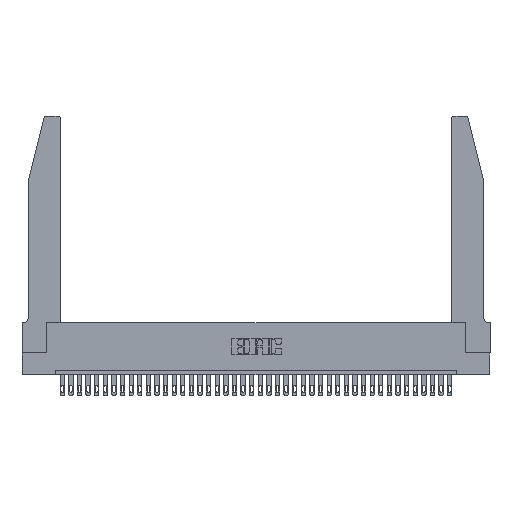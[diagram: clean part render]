
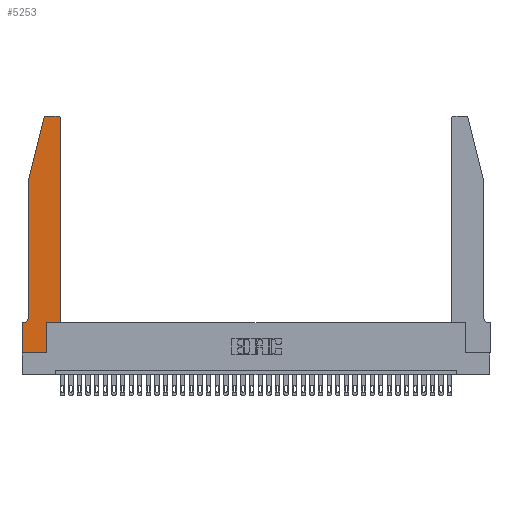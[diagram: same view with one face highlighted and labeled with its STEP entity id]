
A CAD part, top view. The second image highlights one B-rep face of the part: STEP entity #5253.
In plain terms, the highlighted planar face has unit normal (0, 0, 1).
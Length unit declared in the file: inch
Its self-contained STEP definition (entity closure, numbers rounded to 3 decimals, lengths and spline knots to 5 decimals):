
#120 = CARTESIAN_POINT ( 'NONE',  ( 0.2865, 0., 0.37 ) ) ;
#395 = CARTESIAN_POINT ( 'NONE',  ( 0.284, 2.75, 0.37 ) ) ;
#1014 = EDGE_CURVE ( 'NONE', #33882, #28112, #30752, .T. ) ;
#1118 = VERTEX_POINT ( 'NONE', #13074 ) ;
#1124 = LINE ( 'NONE', #24255, #33448 ) ;
#1738 = EDGE_CURVE ( 'NONE', #1118, #33882, #7715, .T. ) ;
#1933 = CARTESIAN_POINT ( 'NONE',  ( 0.2865, 0.35, 0.37 ) ) ;
#1951 = EDGE_LOOP ( 'NONE', ( #24118, #35103, #32265, #30136, #18198, #36965, #20821, #18857, #14239, #2538, #18210, #14275 ) ) ;
#2360 = DIRECTION ( 'NONE',  ( 0., 0., 1. ) ) ;
#2471 = DIRECTION ( 'NONE',  ( 0., -1., 0. ) ) ;
#2538 = ORIENTED_EDGE ( 'NONE', *, *, #29575, .T. ) ;
#2590 = LINE ( 'NONE', #33166, #35360 ) ;
#2778 = VERTEX_POINT ( 'NONE', #35461 ) ;
#3053 = VERTEX_POINT ( 'NONE', #3162 ) ;
#3073 = VECTOR ( 'NONE', #36618, 39.37008 ) ;
#3162 = CARTESIAN_POINT ( 'NONE',  ( 0.0055, 0.35, 0.37 ) ) ;
#3468 = EDGE_CURVE ( 'NONE', #3053, #14425, #10390, .T. ) ;
#3644 = DIRECTION ( 'NONE',  ( -1., 0., 0. ) ) ;
#4509 = CARTESIAN_POINT ( 'NONE',  ( 0.4205, 2.72, 0.37 ) ) ;
#4704 = DIRECTION ( 'NONE',  ( 1., 0., 0. ) ) ;
#5253 = ADVANCED_FACE ( 'NONE', ( #21943 ), #31846, .T. ) ;
#5536 = CARTESIAN_POINT ( 'NONE',  ( 0.2605, 2.75, 0.37 ) ) ;
#5701 = CARTESIAN_POINT ( 'NONE',  ( 0.4505, 0.35, 0.37 ) ) ;
#6025 = LINE ( 'NONE', #5701, #22372 ) ;
#7283 = AXIS2_PLACEMENT_3D ( 'NONE', #8476, #2360, #8876 ) ;
#7715 = LINE ( 'NONE', #5536, #3073 ) ;
#8432 = EDGE_CURVE ( 'NONE', #14425, #2778, #1124, .T. ) ;
#8476 = CARTESIAN_POINT ( 'NONE',  ( 0., 0.35, 0.37 ) ) ;
#8605 = VERTEX_POINT ( 'NONE', #27648 ) ;
#8876 = DIRECTION ( 'NONE',  ( 1., 0., 0. ) ) ;
#9354 = CARTESIAN_POINT ( 'NONE',  ( 0.4505, 2.72, 0.37 ) ) ;
#9806 = EDGE_CURVE ( 'NONE', #36554, #10278, #14082, .T. ) ;
#9826 = VERTEX_POINT ( 'NONE', #35048 ) ;
#10278 = VERTEX_POINT ( 'NONE', #28850 ) ;
#10390 = LINE ( 'NONE', #20717, #37070 ) ;
#10486 = DIRECTION ( 'NONE',  ( 0., 1., 0. ) ) ;
#11458 = DIRECTION ( 'NONE',  ( -1., 0., 0. ) ) ;
#11618 = VERTEX_POINT ( 'NONE', #19619 ) ;
#13074 = CARTESIAN_POINT ( 'NONE',  ( 0.4205, 2.75, 0.37 ) ) ;
#13326 = VECTOR ( 'NONE', #10486, 39.37008 ) ;
#13719 = DIRECTION ( 'NONE',  ( 0., 0., 1. ) ) ;
#14082 = LINE ( 'NONE', #1933, #17372 ) ;
#14101 = EDGE_CURVE ( 'NONE', #9826, #8605, #27517, .T. ) ;
#14239 = ORIENTED_EDGE ( 'NONE', *, *, #9806, .T. ) ;
#14275 = ORIENTED_EDGE ( 'NONE', *, *, #19880, .T. ) ;
#14425 = VERTEX_POINT ( 'NONE', #31439 ) ;
#15294 = EDGE_CURVE ( 'NONE', #2778, #36554, #2590, .T. ) ;
#16641 = LINE ( 'NONE', #32832, #21338 ) ;
#16779 = DIRECTION ( 'NONE',  ( 0., 0., 1. ) ) ;
#17372 = VECTOR ( 'NONE', #37898, 39.37008 ) ;
#18158 = CARTESIAN_POINT ( 'NONE',  ( 0.0055, 0.42, 0.37 ) ) ;
#18198 = ORIENTED_EDGE ( 'NONE', *, *, #27219, .T. ) ;
#18210 = ORIENTED_EDGE ( 'NONE', *, *, #33066, .T. ) ;
#18857 = ORIENTED_EDGE ( 'NONE', *, *, #15294, .T. ) ;
#19619 = CARTESIAN_POINT ( 'NONE',  ( 0.4505, 0.35, 0.37 ) ) ;
#19880 = EDGE_CURVE ( 'NONE', #29419, #1118, #32751, .T. ) ;
#20717 = CARTESIAN_POINT ( 'NONE',  ( 0.0755, 0.35, 0.37 ) ) ;
#20821 = ORIENTED_EDGE ( 'NONE', *, *, #8432, .T. ) ;
#21156 = EDGE_CURVE ( 'NONE', #28112, #9826, #16641, .T. ) ;
#21338 = VECTOR ( 'NONE', #30619, 39.37008 ) ;
#21943 = FACE_OUTER_BOUND ( 'NONE', #1951, .T. ) ;
#21995 = CARTESIAN_POINT ( 'NONE',  ( 0.284, 2.72, 0.37 ) ) ;
#22372 = VECTOR ( 'NONE', #29413, 39.37008 ) ;
#22540 = AXIS2_PLACEMENT_3D ( 'NONE', #18158, #27367, #3644 ) ;
#24118 = ORIENTED_EDGE ( 'NONE', *, *, #1738, .T. ) ;
#24255 = CARTESIAN_POINT ( 'NONE',  ( 0., 0., 0.37 ) ) ;
#25555 = DIRECTION ( 'NONE',  ( 1., 0., 0. ) ) ;
#25920 = CARTESIAN_POINT ( 'NONE',  ( 0.0755, 2., 0.37 ) ) ;
#26190 = DIRECTION ( 'NONE',  ( 0., -1., 0. ) ) ;
#27054 = VECTOR ( 'NONE', #26190, 39.37008 ) ;
#27219 = EDGE_CURVE ( 'NONE', #8605, #3053, #35181, .T. ) ;
#27367 = DIRECTION ( 'NONE',  ( 0., 0., -1. ) ) ;
#27517 = LINE ( 'NONE', #25920, #27054 ) ;
#27648 = CARTESIAN_POINT ( 'NONE',  ( 0.0755, 0.42, 0.37 ) ) ;
#28112 = VERTEX_POINT ( 'NONE', #38316 ) ;
#28827 = CARTESIAN_POINT ( 'NONE',  ( 0.4505, 0.35, 0.37 ) ) ;
#28850 = CARTESIAN_POINT ( 'NONE',  ( 0.2865, 0.35, 0.37 ) ) ;
#29358 = LINE ( 'NONE', #28827, #13326 ) ;
#29413 = DIRECTION ( 'NONE',  ( 1., 0., 0. ) ) ;
#29419 = VERTEX_POINT ( 'NONE', #9354 ) ;
#29575 = EDGE_CURVE ( 'NONE', #10278, #11618, #6025, .T. ) ;
#30136 = ORIENTED_EDGE ( 'NONE', *, *, #14101, .T. ) ;
#30452 = AXIS2_PLACEMENT_3D ( 'NONE', #4509, #16779, #31786 ) ;
#30619 = DIRECTION ( 'NONE',  ( -0.239, -0.971, 0. ) ) ;
#30752 = CIRCLE ( 'NONE', #31321, 0.03 ) ;
#31321 = AXIS2_PLACEMENT_3D ( 'NONE', #21995, #13719, #4704 ) ;
#31439 = CARTESIAN_POINT ( 'NONE',  ( 0., 0.35, 0.37 ) ) ;
#31786 = DIRECTION ( 'NONE',  ( 1., 0., 0. ) ) ;
#31846 = PLANE ( 'NONE',  #7283 ) ;
#32265 = ORIENTED_EDGE ( 'NONE', *, *, #21156, .T. ) ;
#32751 = CIRCLE ( 'NONE', #30452, 0.03 ) ;
#32832 = CARTESIAN_POINT ( 'NONE',  ( 0.0755, 2., 0.37 ) ) ;
#33066 = EDGE_CURVE ( 'NONE', #11618, #29419, #29358, .T. ) ;
#33166 = CARTESIAN_POINT ( 'NONE',  ( 0., 0., 0.37 ) ) ;
#33448 = VECTOR ( 'NONE', #2471, 39.37008 ) ;
#33882 = VERTEX_POINT ( 'NONE', #395 ) ;
#35048 = CARTESIAN_POINT ( 'NONE',  ( 0.0755, 2., 0.37 ) ) ;
#35103 = ORIENTED_EDGE ( 'NONE', *, *, #1014, .T. ) ;
#35181 = CIRCLE ( 'NONE', #22540, 0.07 ) ;
#35360 = VECTOR ( 'NONE', #25555, 39.37008 ) ;
#35461 = CARTESIAN_POINT ( 'NONE',  ( 0., 0., 0.37 ) ) ;
#36554 = VERTEX_POINT ( 'NONE', #120 ) ;
#36618 = DIRECTION ( 'NONE',  ( -1., 0., 0. ) ) ;
#36965 = ORIENTED_EDGE ( 'NONE', *, *, #3468, .T. ) ;
#37070 = VECTOR ( 'NONE', #11458, 39.37008 ) ;
#37898 = DIRECTION ( 'NONE',  ( 0., 1., 0. ) ) ;
#38316 = CARTESIAN_POINT ( 'NONE',  ( 0.25487, 2.72718, 0.37 ) ) ;
